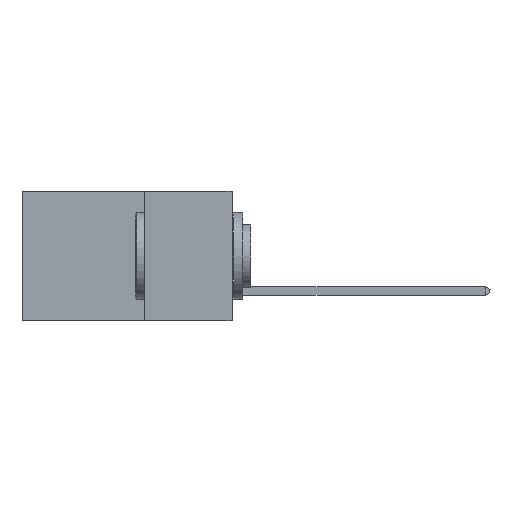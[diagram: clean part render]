
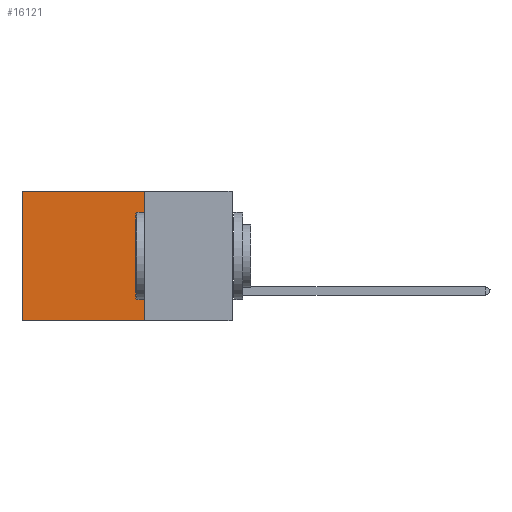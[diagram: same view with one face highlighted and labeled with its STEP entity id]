
A CAD part, left-side view. The second image highlights one B-rep face of the part: STEP entity #16121.
In plain terms, the highlighted planar face has unit normal (-1, 0, 0).
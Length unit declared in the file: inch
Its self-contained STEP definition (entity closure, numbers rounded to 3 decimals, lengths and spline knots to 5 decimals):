
#39 = VECTOR ( 'NONE', #13162, 39.37008 ) ;
#420 = VERTEX_POINT ( 'NONE', #1396 ) ;
#745 = PLANE ( 'NONE',  #15463 ) ;
#1090 = CARTESIAN_POINT ( 'NONE',  ( 0.2875, 0.6, 0. ) ) ;
#1396 = CARTESIAN_POINT ( 'NONE',  ( 0.2875, 0.6, 0. ) ) ;
#2029 = EDGE_CURVE ( 'NONE', #4216, #420, #15843, .T. ) ;
#2829 = LINE ( 'NONE', #11772, #6105 ) ;
#3636 = VECTOR ( 'NONE', #5866, 39.37008 ) ;
#4210 = CARTESIAN_POINT ( 'NONE',  ( 0.2875, 0.25, 0. ) ) ;
#4216 = VERTEX_POINT ( 'NONE', #14953 ) ;
#4345 = ORIENTED_EDGE ( 'NONE', *, *, #9320, .F. ) ;
#4621 = LINE ( 'NONE', #8932, #39 ) ;
#4909 = DIRECTION ( 'NONE',  ( 0., 0., -1. ) ) ;
#5302 = EDGE_CURVE ( 'NONE', #420, #8427, #15918, .T. ) ;
#5624 = ORIENTED_EDGE ( 'NONE', *, *, #2029, .T. ) ;
#5650 = VERTEX_POINT ( 'NONE', #12727 ) ;
#5866 = DIRECTION ( 'NONE',  ( 0., 1., 0. ) ) ;
#6105 = VECTOR ( 'NONE', #11586, 39.37008 ) ;
#8194 = DIRECTION ( 'NONE',  ( 0., 0., -1. ) ) ;
#8427 = VERTEX_POINT ( 'NONE', #13563 ) ;
#8710 = ORIENTED_EDGE ( 'NONE', *, *, #5302, .T. ) ;
#8932 = CARTESIAN_POINT ( 'NONE',  ( 0.2875, 0.25, -0.37 ) ) ;
#9320 = EDGE_CURVE ( 'NONE', #4216, #5650, #2829, .T. ) ;
#10691 = VECTOR ( 'NONE', #8194, 39.37008 ) ;
#11586 = DIRECTION ( 'NONE',  ( 0., 0., -1. ) ) ;
#11772 = CARTESIAN_POINT ( 'NONE',  ( 0.2875, 0.25, 0. ) ) ;
#12120 = CARTESIAN_POINT ( 'NONE',  ( 0.2875, 0.25, 0. ) ) ;
#12727 = CARTESIAN_POINT ( 'NONE',  ( 0.2875, 0.25, -0.37 ) ) ;
#13039 = EDGE_LOOP ( 'NONE', ( #8710, #16141, #4345, #5624 ) ) ;
#13162 = DIRECTION ( 'NONE',  ( 0., 1., 0. ) ) ;
#13563 = CARTESIAN_POINT ( 'NONE',  ( 0.2875, 0.6, -0.37 ) ) ;
#14953 = CARTESIAN_POINT ( 'NONE',  ( 0.2875, 0.25, 0. ) ) ;
#14964 = FACE_OUTER_BOUND ( 'NONE', #13039, .T. ) ;
#15463 = AXIS2_PLACEMENT_3D ( 'NONE', #12120, #16245, #4909 ) ;
#15843 = LINE ( 'NONE', #4210, #3636 ) ;
#15918 = LINE ( 'NONE', #1090, #10691 ) ;
#16121 = ADVANCED_FACE ( 'NONE', ( #14964 ), #745, .F. ) ;
#16141 = ORIENTED_EDGE ( 'NONE', *, *, #17884, .F. ) ;
#16245 = DIRECTION ( 'NONE',  ( 1., 0., 0. ) ) ;
#17884 = EDGE_CURVE ( 'NONE', #5650, #8427, #4621, .T. ) ;
